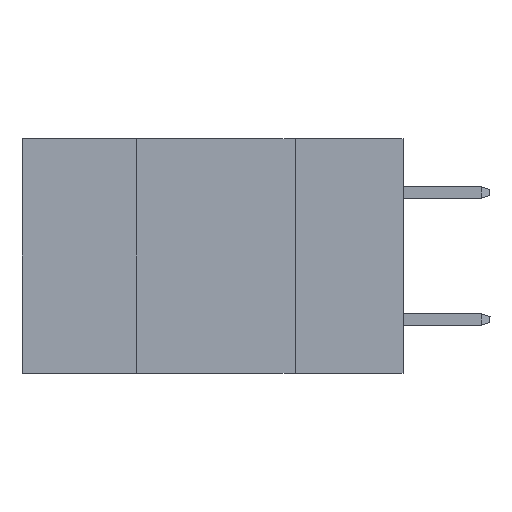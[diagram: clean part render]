
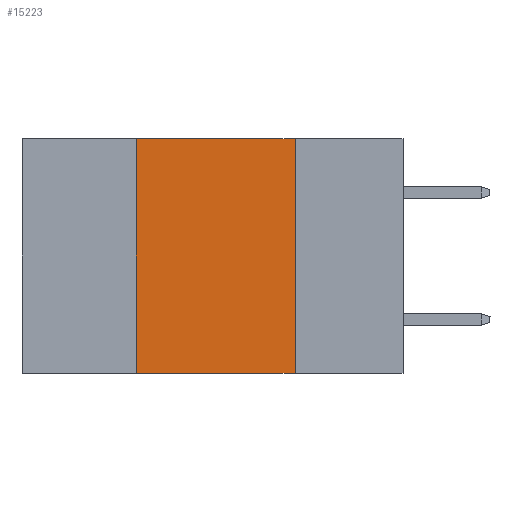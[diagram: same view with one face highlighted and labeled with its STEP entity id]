
A CAD part, left-side view. The second image highlights one B-rep face of the part: STEP entity #15223.
In plain terms, the highlighted planar face has unit normal (-1, 0, 0).
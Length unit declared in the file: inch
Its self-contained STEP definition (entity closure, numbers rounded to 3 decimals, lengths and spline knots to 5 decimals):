
#546 = EDGE_LOOP ( 'NONE', ( #10779, #12148, #13168, #5733 ) ) ;
#1921 = VECTOR ( 'NONE', #5421, 39.37008 ) ;
#1983 = EDGE_CURVE ( 'NONE', #5230, #2932, #4026, .T. ) ;
#2450 = EDGE_CURVE ( 'NONE', #11562, #5230, #14341, .T. ) ;
#2641 = CARTESIAN_POINT ( 'NONE',  ( 0., 0.6, 0. ) ) ;
#2932 = VERTEX_POINT ( 'NONE', #6094 ) ;
#3355 = CARTESIAN_POINT ( 'NONE',  ( 0., 0.6, -0.37 ) ) ;
#3432 = VECTOR ( 'NONE', #7249, 39.37008 ) ;
#4026 = LINE ( 'NONE', #4112, #8203 ) ;
#4043 = DIRECTION ( 'NONE',  ( 1., 0., 0. ) ) ;
#4112 = CARTESIAN_POINT ( 'NONE',  ( 0., 0.17, 0. ) ) ;
#5230 = VERTEX_POINT ( 'NONE', #14727 ) ;
#5421 = DIRECTION ( 'NONE',  ( 0., -1., 0. ) ) ;
#5733 = ORIENTED_EDGE ( 'NONE', *, *, #6806, .T. ) ;
#6094 = CARTESIAN_POINT ( 'NONE',  ( 0., 0.17, -0.37 ) ) ;
#6114 = CARTESIAN_POINT ( 'NONE',  ( 0., 0.42, 0. ) ) ;
#6806 = EDGE_CURVE ( 'NONE', #13388, #2932, #13665, .T. ) ;
#6937 = CARTESIAN_POINT ( 'NONE',  ( 0., 0.42, -0.37 ) ) ;
#7249 = DIRECTION ( 'NONE',  ( 0., 0., 1. ) ) ;
#7326 = LINE ( 'NONE', #16643, #3432 ) ;
#7913 = EDGE_CURVE ( 'NONE', #13388, #11562, #7326, .T. ) ;
#8133 = AXIS2_PLACEMENT_3D ( 'NONE', #2641, #4043, #15406 ) ;
#8203 = VECTOR ( 'NONE', #13199, 39.37008 ) ;
#10779 = ORIENTED_EDGE ( 'NONE', *, *, #1983, .F. ) ;
#11461 = FACE_OUTER_BOUND ( 'NONE', #546, .T. ) ;
#11562 = VERTEX_POINT ( 'NONE', #6114 ) ;
#12148 = ORIENTED_EDGE ( 'NONE', *, *, #2450, .F. ) ;
#12919 = CARTESIAN_POINT ( 'NONE',  ( 0., 0.6, 0. ) ) ;
#13168 = ORIENTED_EDGE ( 'NONE', *, *, #7913, .F. ) ;
#13199 = DIRECTION ( 'NONE',  ( 0., 0., -1. ) ) ;
#13388 = VERTEX_POINT ( 'NONE', #6937 ) ;
#13665 = LINE ( 'NONE', #3355, #13753 ) ;
#13753 = VECTOR ( 'NONE', #16435, 39.37008 ) ;
#14135 = PLANE ( 'NONE',  #8133 ) ;
#14341 = LINE ( 'NONE', #12919, #1921 ) ;
#14727 = CARTESIAN_POINT ( 'NONE',  ( 0., 0.17, 0. ) ) ;
#15223 = ADVANCED_FACE ( 'NONE', ( #11461 ), #14135, .F. ) ;
#15406 = DIRECTION ( 'NONE',  ( 0., 0., -1. ) ) ;
#16435 = DIRECTION ( 'NONE',  ( 0., -1., 0. ) ) ;
#16643 = CARTESIAN_POINT ( 'NONE',  ( 0., 0.42, 0. ) ) ;
